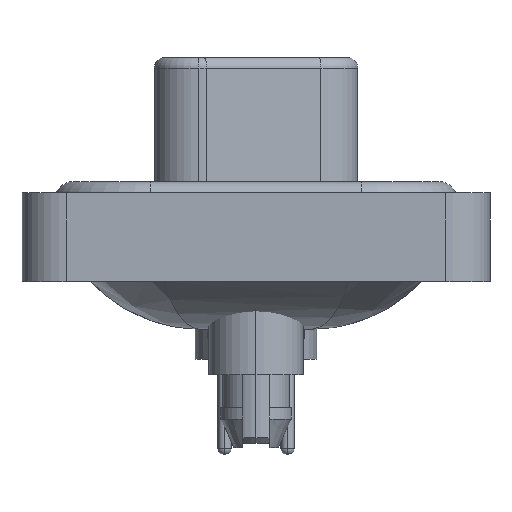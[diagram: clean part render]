
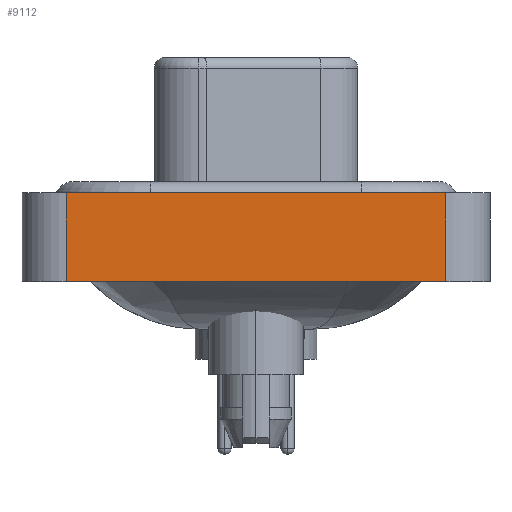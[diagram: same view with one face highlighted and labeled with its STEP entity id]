
A CAD part, left-side view. The second image highlights one B-rep face of the part: STEP entity #9112.
In plain terms, the highlighted planar face has unit normal (-1, 0, 0).
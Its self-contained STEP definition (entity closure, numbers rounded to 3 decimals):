
#313 = VECTOR ( 'NONE', #19804, 1000. ) ;
#3069 = PLANE ( 'NONE',  #10915 ) ;
#3148 = DIRECTION ( 'NONE',  ( 0., 0., 1. ) ) ;
#4834 = LINE ( 'NONE', #11950, #20504 ) ;
#4918 = VERTEX_POINT ( 'NONE', #14245 ) ;
#5605 = CARTESIAN_POINT ( 'NONE',  ( -7.25, -8.55, -3.6 ) ) ;
#6248 = VECTOR ( 'NONE', #3148, 1000. ) ;
#6545 = DIRECTION ( 'NONE',  ( 0., 0., 1. ) ) ;
#6658 = EDGE_CURVE ( 'NONE', #13502, #17248, #19330, .T. ) ;
#7779 = CARTESIAN_POINT ( 'NONE',  ( -7.25, -8.55, -3.6 ) ) ;
#8534 = LINE ( 'NONE', #18711, #6248 ) ;
#9036 = DIRECTION ( 'NONE',  ( 0., -1., 0. ) ) ;
#9112 = ADVANCED_FACE ( 'NONE', ( #11786 ), #3069, .T. ) ;
#10915 = AXIS2_PLACEMENT_3D ( 'NONE', #7779, #14772, #21744 ) ;
#11035 = EDGE_CURVE ( 'NONE', #17248, #12272, #8534, .T. ) ;
#11714 = EDGE_CURVE ( 'NONE', #4918, #12272, #14561, .T. ) ;
#11786 = FACE_OUTER_BOUND ( 'NONE', #15441, .T. ) ;
#11950 = CARTESIAN_POINT ( 'NONE',  ( -7.25, 8.55, -3.6 ) ) ;
#12272 = VERTEX_POINT ( 'NONE', #13565 ) ;
#12852 = ORIENTED_EDGE ( 'NONE', *, *, #11035, .T. ) ;
#13502 = VERTEX_POINT ( 'NONE', #16462 ) ;
#13565 = CARTESIAN_POINT ( 'NONE',  ( -7.25, -8.55, 0.4 ) ) ;
#14038 = EDGE_CURVE ( 'NONE', #13502, #4918, #4834, .T. ) ;
#14245 = CARTESIAN_POINT ( 'NONE',  ( -7.25, 8.55, 0.4 ) ) ;
#14561 = LINE ( 'NONE', #20027, #313 ) ;
#14772 = DIRECTION ( 'NONE',  ( -1., 0., 0. ) ) ;
#15208 = CARTESIAN_POINT ( 'NONE',  ( -7.25, -8.55, -3.6 ) ) ;
#15441 = EDGE_LOOP ( 'NONE', ( #12852, #17369, #20859, #22600 ) ) ;
#16462 = CARTESIAN_POINT ( 'NONE',  ( -7.25, 8.55, -3.6 ) ) ;
#17248 = VERTEX_POINT ( 'NONE', #15208 ) ;
#17369 = ORIENTED_EDGE ( 'NONE', *, *, #11714, .F. ) ;
#18711 = CARTESIAN_POINT ( 'NONE',  ( -7.25, -8.55, -3.6 ) ) ;
#19214 = VECTOR ( 'NONE', #9036, 1000. ) ;
#19330 = LINE ( 'NONE', #5605, #19214 ) ;
#19804 = DIRECTION ( 'NONE',  ( 0., -1., 0. ) ) ;
#20027 = CARTESIAN_POINT ( 'NONE',  ( -7.25, -8.55, 0.4 ) ) ;
#20504 = VECTOR ( 'NONE', #6545, 1000. ) ;
#20859 = ORIENTED_EDGE ( 'NONE', *, *, #14038, .F. ) ;
#21744 = DIRECTION ( 'NONE',  ( 0., 0., 1. ) ) ;
#22600 = ORIENTED_EDGE ( 'NONE', *, *, #6658, .T. ) ;
